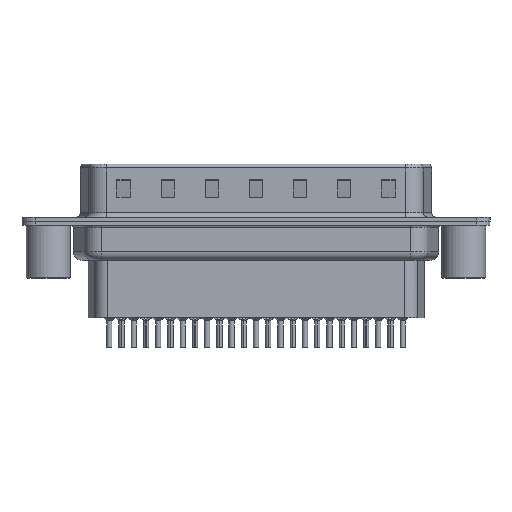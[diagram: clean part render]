
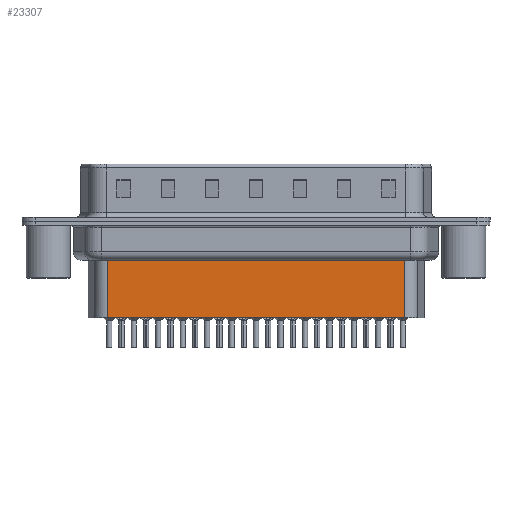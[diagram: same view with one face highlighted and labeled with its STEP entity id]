
A CAD part, front view. The second image highlights one B-rep face of the part: STEP entity #23307.
In plain terms, the highlighted planar face has unit normal (0, -1, 0).
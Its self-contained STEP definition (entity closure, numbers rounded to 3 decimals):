
#221 = VERTEX_POINT ( 'NONE', #9038 ) ;
#1455 = CARTESIAN_POINT ( 'NONE',  ( 6.706, -3.5, -3.1 ) ) ;
#1790 = CARTESIAN_POINT ( 'NONE',  ( 6.706, -3.5, -10.95 ) ) ;
#2194 = CARTESIAN_POINT ( 'NONE',  ( 6.706, -3.5, -10.95 ) ) ;
#3329 = AXIS2_PLACEMENT_3D ( 'NONE', #16840, #10742, #10988 ) ;
#4791 = EDGE_CURVE ( 'NONE', #11013, #9663, #15090, .T. ) ;
#4841 = DIRECTION ( 'NONE',  ( 0., 0., -1. ) ) ;
#6532 = CARTESIAN_POINT ( 'NONE',  ( 40.344, -3.5, -3.1 ) ) ;
#6940 = ORIENTED_EDGE ( 'NONE', *, *, #23691, .F. ) ;
#6950 = ORIENTED_EDGE ( 'NONE', *, *, #13306, .T. ) ;
#6966 = VECTOR ( 'NONE', #17592, 1000. ) ;
#7050 = LINE ( 'NONE', #6532, #12828 ) ;
#7092 = VECTOR ( 'NONE', #23431, 1000. ) ;
#7921 = CARTESIAN_POINT ( 'NONE',  ( 6.459, -3.5, -4.097 ) ) ;
#9038 = CARTESIAN_POINT ( 'NONE',  ( 40.344, -3.5, -4.097 ) ) ;
#9663 = VERTEX_POINT ( 'NONE', #2194 ) ;
#9831 = LINE ( 'NONE', #1790, #22077 ) ;
#10024 = EDGE_CURVE ( 'NONE', #11223, #9663, #9831, .T. ) ;
#10742 = DIRECTION ( 'NONE',  ( 0., -1., 0. ) ) ;
#10988 = DIRECTION ( 'NONE',  ( 1., 0., 0. ) ) ;
#11013 = VERTEX_POINT ( 'NONE', #23979 ) ;
#11223 = VERTEX_POINT ( 'NONE', #20705 ) ;
#12828 = VECTOR ( 'NONE', #4841, 1000. ) ;
#13306 = EDGE_CURVE ( 'NONE', #221, #11013, #13674, .T. ) ;
#13674 = LINE ( 'NONE', #7921, #6966 ) ;
#15090 = LINE ( 'NONE', #1455, #7092 ) ;
#16708 = PLANE ( 'NONE',  #3329 ) ;
#16840 = CARTESIAN_POINT ( 'NONE',  ( 6.706, -3.5, -3.1 ) ) ;
#17164 = EDGE_LOOP ( 'NONE', ( #6940, #6950, #23077, #22403 ) ) ;
#17592 = DIRECTION ( 'NONE',  ( -1., 0., 0. ) ) ;
#18012 = DIRECTION ( 'NONE',  ( -1., 0., 0. ) ) ;
#20705 = CARTESIAN_POINT ( 'NONE',  ( 40.344, -3.5, -10.95 ) ) ;
#20761 = FACE_OUTER_BOUND ( 'NONE', #17164, .T. ) ;
#22077 = VECTOR ( 'NONE', #18012, 1000. ) ;
#22403 = ORIENTED_EDGE ( 'NONE', *, *, #10024, .F. ) ;
#23077 = ORIENTED_EDGE ( 'NONE', *, *, #4791, .T. ) ;
#23307 = ADVANCED_FACE ( 'NONE', ( #20761 ), #16708, .T. ) ;
#23431 = DIRECTION ( 'NONE',  ( 0., 0., -1. ) ) ;
#23691 = EDGE_CURVE ( 'NONE', #221, #11223, #7050, .T. ) ;
#23979 = CARTESIAN_POINT ( 'NONE',  ( 6.706, -3.5, -4.097 ) ) ;
